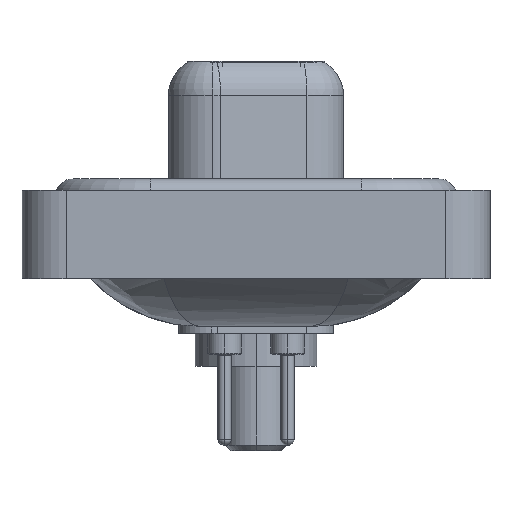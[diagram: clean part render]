
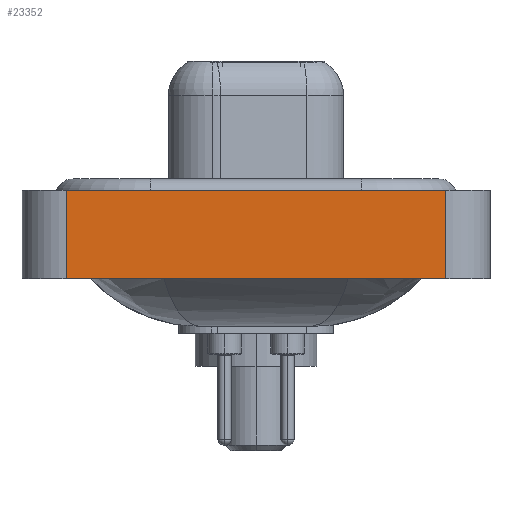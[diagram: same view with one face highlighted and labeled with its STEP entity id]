
A CAD part, left-side view. The second image highlights one B-rep face of the part: STEP entity #23352.
In plain terms, the highlighted planar face has unit normal (-1, 0, 0).
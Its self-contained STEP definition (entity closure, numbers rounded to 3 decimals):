
#30 = LINE ( 'NONE', #22594, #24008 ) ;
#104 = EDGE_CURVE ( 'NONE', #23400, #24331, #30, .T. ) ;
#2395 = CARTESIAN_POINT ( 'NONE',  ( -7.35, -8.55, -3.6 ) ) ;
#2612 = EDGE_CURVE ( 'NONE', #6730, #23400, #12377, .T. ) ;
#4246 = FACE_OUTER_BOUND ( 'NONE', #10541, .T. ) ;
#4546 = LINE ( 'NONE', #14607, #10598 ) ;
#5328 = ORIENTED_EDGE ( 'NONE', *, *, #20743, .T. ) ;
#6526 = CARTESIAN_POINT ( 'NONE',  ( -7.35, 8.55, 0.4 ) ) ;
#6730 = VERTEX_POINT ( 'NONE', #14012 ) ;
#7969 = VERTEX_POINT ( 'NONE', #17230 ) ;
#8505 = VECTOR ( 'NONE', #16872, 1000. ) ;
#10053 = DIRECTION ( 'NONE',  ( 0., -1., 0. ) ) ;
#10437 = DIRECTION ( 'NONE',  ( 0., 0., 1. ) ) ;
#10541 = EDGE_LOOP ( 'NONE', ( #5328, #15420, #12634, #11598 ) ) ;
#10598 = VECTOR ( 'NONE', #18828, 1000. ) ;
#11579 = LINE ( 'NONE', #23575, #24764 ) ;
#11598 = ORIENTED_EDGE ( 'NONE', *, *, #16875, .T. ) ;
#12174 = DIRECTION ( 'NONE',  ( -1., 0., 0. ) ) ;
#12377 = LINE ( 'NONE', #20429, #8505 ) ;
#12634 = ORIENTED_EDGE ( 'NONE', *, *, #2612, .F. ) ;
#14012 = CARTESIAN_POINT ( 'NONE',  ( -7.35, 8.55, -3.6 ) ) ;
#14607 = CARTESIAN_POINT ( 'NONE',  ( -7.35, -8.55, -3.6 ) ) ;
#15294 = CARTESIAN_POINT ( 'NONE',  ( -7.35, -8.55, 0.4 ) ) ;
#15420 = ORIENTED_EDGE ( 'NONE', *, *, #104, .F. ) ;
#16872 = DIRECTION ( 'NONE',  ( 0., 0., 1. ) ) ;
#16875 = EDGE_CURVE ( 'NONE', #6730, #7969, #4546, .T. ) ;
#17230 = CARTESIAN_POINT ( 'NONE',  ( -7.35, -8.55, -3.6 ) ) ;
#18828 = DIRECTION ( 'NONE',  ( 0., -1., 0. ) ) ;
#20353 = PLANE ( 'NONE',  #21483 ) ;
#20429 = CARTESIAN_POINT ( 'NONE',  ( -7.35, 8.55, -3.6 ) ) ;
#20743 = EDGE_CURVE ( 'NONE', #7969, #24331, #11579, .T. ) ;
#21483 = AXIS2_PLACEMENT_3D ( 'NONE', #2395, #12174, #10437 ) ;
#21738 = DIRECTION ( 'NONE',  ( 0., 0., 1. ) ) ;
#22594 = CARTESIAN_POINT ( 'NONE',  ( -7.35, -8.55, 0.4 ) ) ;
#23352 = ADVANCED_FACE ( 'NONE', ( #4246 ), #20353, .T. ) ;
#23400 = VERTEX_POINT ( 'NONE', #6526 ) ;
#23575 = CARTESIAN_POINT ( 'NONE',  ( -7.35, -8.55, -3.6 ) ) ;
#24008 = VECTOR ( 'NONE', #10053, 1000. ) ;
#24331 = VERTEX_POINT ( 'NONE', #15294 ) ;
#24764 = VECTOR ( 'NONE', #21738, 1000. ) ;
